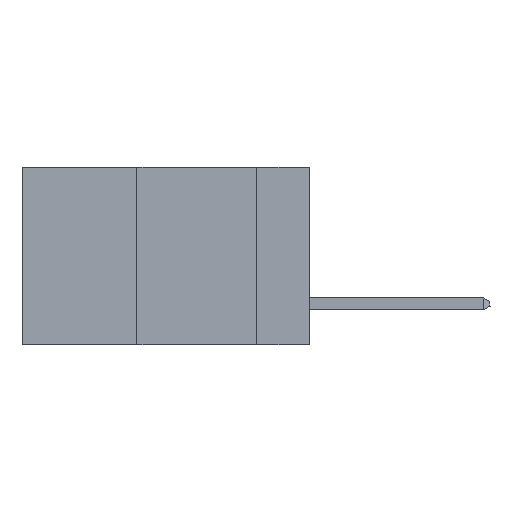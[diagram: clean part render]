
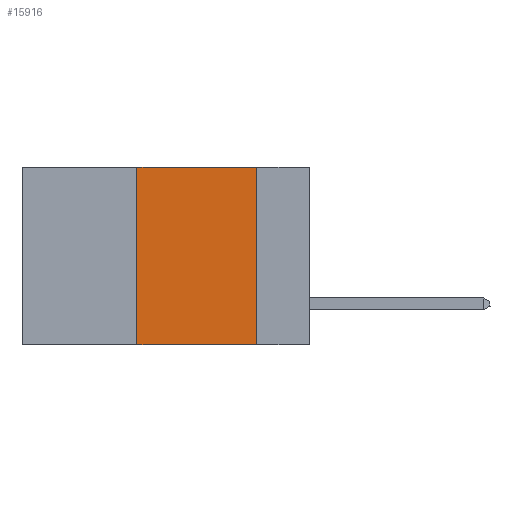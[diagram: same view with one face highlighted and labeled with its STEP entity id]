
A CAD part, left-side view. The second image highlights one B-rep face of the part: STEP entity #15916.
In plain terms, the highlighted planar face has unit normal (-1, 0, 0).
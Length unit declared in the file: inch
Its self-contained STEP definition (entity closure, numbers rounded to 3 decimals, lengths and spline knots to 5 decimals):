
#3055 = CARTESIAN_POINT ( 'NONE',  ( 0., 0.11, 0. ) ) ;
#4540 = DIRECTION ( 'NONE',  ( 1., 0., 0. ) ) ;
#6320 = DIRECTION ( 'NONE',  ( 0., 0., -1. ) ) ;
#6462 = FACE_OUTER_BOUND ( 'NONE', #9551, .T. ) ;
#6642 = ORIENTED_EDGE ( 'NONE', *, *, #12418, .F. ) ;
#9551 = EDGE_LOOP ( 'NONE', ( #6642, #15131, #31878, #13987 ) ) ;
#9732 = LINE ( 'NONE', #42297, #33705 ) ;
#12418 = EDGE_CURVE ( 'NONE', #24436, #43181, #16735, .T. ) ;
#12478 = DIRECTION ( 'NONE',  ( 0., 0., 1. ) ) ;
#13007 = VECTOR ( 'NONE', #20902, 39.37008 ) ;
#13987 = ORIENTED_EDGE ( 'NONE', *, *, #34357, .T. ) ;
#14734 = EDGE_CURVE ( 'NONE', #37270, #39883, #27726, .T. ) ;
#15131 = ORIENTED_EDGE ( 'NONE', *, *, #32496, .F. ) ;
#15330 = CARTESIAN_POINT ( 'NONE',  ( 0., 0.36, 0. ) ) ;
#15916 = ADVANCED_FACE ( 'NONE', ( #6462 ), #21090, .F. ) ;
#16735 = LINE ( 'NONE', #3055, #28503 ) ;
#18244 = CARTESIAN_POINT ( 'NONE',  ( 0., 0.6, 0. ) ) ;
#19578 = CARTESIAN_POINT ( 'NONE',  ( 0., 0.11, 0. ) ) ;
#20902 = DIRECTION ( 'NONE',  ( 0., -1., 0. ) ) ;
#21090 = PLANE ( 'NONE',  #28687 ) ;
#22670 = LINE ( 'NONE', #27355, #13007 ) ;
#23780 = CARTESIAN_POINT ( 'NONE',  ( 0., 0.36, -0.37 ) ) ;
#24436 = VERTEX_POINT ( 'NONE', #19578 ) ;
#26153 = VECTOR ( 'NONE', #12478, 39.37008 ) ;
#26506 = CARTESIAN_POINT ( 'NONE',  ( 0., 0.11, -0.37 ) ) ;
#27355 = CARTESIAN_POINT ( 'NONE',  ( 0., 0.6, 0. ) ) ;
#27726 = LINE ( 'NONE', #15330, #26153 ) ;
#28503 = VECTOR ( 'NONE', #6320, 39.37008 ) ;
#28687 = AXIS2_PLACEMENT_3D ( 'NONE', #18244, #4540, #42036 ) ;
#31878 = ORIENTED_EDGE ( 'NONE', *, *, #14734, .F. ) ;
#32496 = EDGE_CURVE ( 'NONE', #39883, #24436, #22670, .T. ) ;
#33705 = VECTOR ( 'NONE', #41704, 39.37008 ) ;
#34357 = EDGE_CURVE ( 'NONE', #37270, #43181, #9732, .T. ) ;
#37270 = VERTEX_POINT ( 'NONE', #23780 ) ;
#39883 = VERTEX_POINT ( 'NONE', #42650 ) ;
#41704 = DIRECTION ( 'NONE',  ( 0., -1., 0. ) ) ;
#42036 = DIRECTION ( 'NONE',  ( 0., 0., -1. ) ) ;
#42297 = CARTESIAN_POINT ( 'NONE',  ( 0., 0.6, -0.37 ) ) ;
#42650 = CARTESIAN_POINT ( 'NONE',  ( 0., 0.36, 0. ) ) ;
#43181 = VERTEX_POINT ( 'NONE', #26506 ) ;
